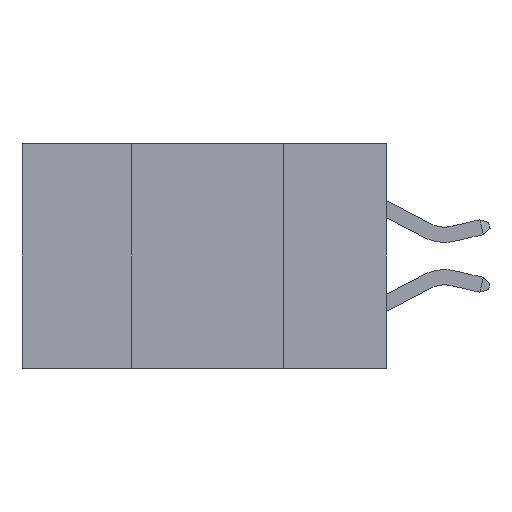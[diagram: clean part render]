
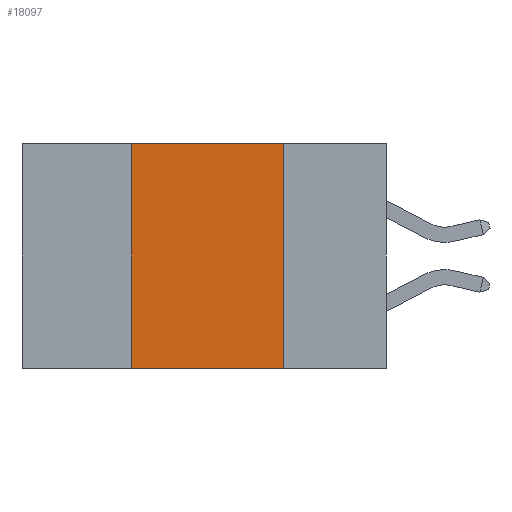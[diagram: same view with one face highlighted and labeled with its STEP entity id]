
A CAD part, left-side view. The second image highlights one B-rep face of the part: STEP entity #18097.
In plain terms, the highlighted planar face has unit normal (-1, 0, 0).
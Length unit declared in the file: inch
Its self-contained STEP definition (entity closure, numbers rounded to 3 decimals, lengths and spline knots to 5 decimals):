
#22 = CARTESIAN_POINT ( 'NONE',  ( 0., 0.17, 0. ) ) ;
#313 = LINE ( 'NONE', #6578, #3722 ) ;
#1223 = CARTESIAN_POINT ( 'NONE',  ( 0., 0.42, 0. ) ) ;
#1805 = CARTESIAN_POINT ( 'NONE',  ( 0., 0.42, -0.37 ) ) ;
#2480 = LINE ( 'NONE', #20772, #18701 ) ;
#2529 = ORIENTED_EDGE ( 'NONE', *, *, #25284, .T. ) ;
#3722 = VECTOR ( 'NONE', #12074, 39.37008 ) ;
#4099 = AXIS2_PLACEMENT_3D ( 'NONE', #15795, #13904, #23938 ) ;
#5253 = ORIENTED_EDGE ( 'NONE', *, *, #6351, .F. ) ;
#5258 = LINE ( 'NONE', #17284, #17796 ) ;
#6351 = EDGE_CURVE ( 'NONE', #9457, #12600, #22102, .T. ) ;
#6578 = CARTESIAN_POINT ( 'NONE',  ( 0., 0.6, -0.37 ) ) ;
#7672 = ORIENTED_EDGE ( 'NONE', *, *, #9584, .F. ) ;
#9131 = DIRECTION ( 'NONE',  ( 0., -1., 0. ) ) ;
#9457 = VERTEX_POINT ( 'NONE', #23148 ) ;
#9584 = EDGE_CURVE ( 'NONE', #12600, #16798, #5258, .T. ) ;
#10050 = PLANE ( 'NONE',  #4099 ) ;
#12074 = DIRECTION ( 'NONE',  ( 0., -1., 0. ) ) ;
#12600 = VERTEX_POINT ( 'NONE', #1223 ) ;
#13904 = DIRECTION ( 'NONE',  ( 1., 0., 0. ) ) ;
#14890 = DIRECTION ( 'NONE',  ( 0., 0., -1. ) ) ;
#15795 = CARTESIAN_POINT ( 'NONE',  ( 0., 0.6, 0. ) ) ;
#15903 = EDGE_CURVE ( 'NONE', #16798, #23411, #2480, .T. ) ;
#16798 = VERTEX_POINT ( 'NONE', #22 ) ;
#17284 = CARTESIAN_POINT ( 'NONE',  ( 0., 0.6, 0. ) ) ;
#17796 = VECTOR ( 'NONE', #9131, 39.37008 ) ;
#18097 = ADVANCED_FACE ( 'NONE', ( #22197 ), #10050, .F. ) ;
#18197 = VECTOR ( 'NONE', #24245, 39.37008 ) ;
#18701 = VECTOR ( 'NONE', #14890, 39.37008 ) ;
#18984 = EDGE_LOOP ( 'NONE', ( #22573, #7672, #5253, #2529 ) ) ;
#19810 = CARTESIAN_POINT ( 'NONE',  ( 0., 0.17, -0.37 ) ) ;
#20772 = CARTESIAN_POINT ( 'NONE',  ( 0., 0.17, -0.37 ) ) ;
#22102 = LINE ( 'NONE', #1805, #18197 ) ;
#22197 = FACE_OUTER_BOUND ( 'NONE', #18984, .T. ) ;
#22573 = ORIENTED_EDGE ( 'NONE', *, *, #15903, .F. ) ;
#23148 = CARTESIAN_POINT ( 'NONE',  ( 0., 0.42, -0.37 ) ) ;
#23411 = VERTEX_POINT ( 'NONE', #19810 ) ;
#23938 = DIRECTION ( 'NONE',  ( 0., 0., -1. ) ) ;
#24245 = DIRECTION ( 'NONE',  ( 0., 0., 1. ) ) ;
#25284 = EDGE_CURVE ( 'NONE', #9457, #23411, #313, .T. ) ;
